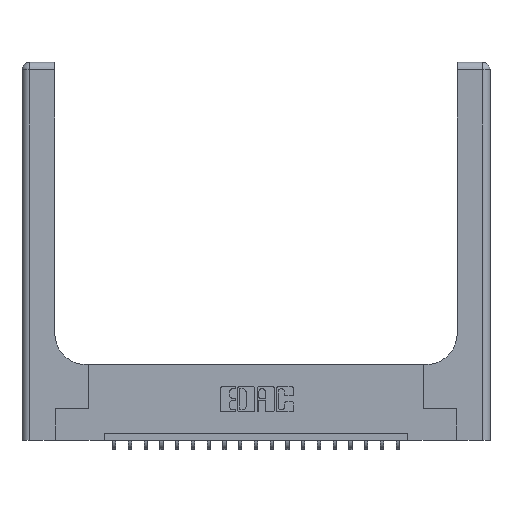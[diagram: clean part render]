
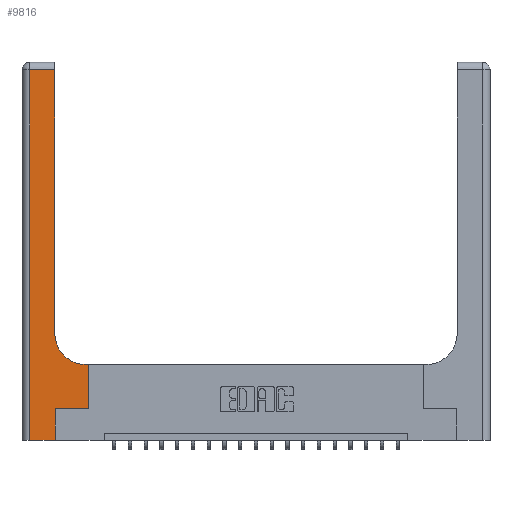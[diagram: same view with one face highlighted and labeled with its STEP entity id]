
A CAD part, top view. The second image highlights one B-rep face of the part: STEP entity #9816.
In plain terms, the highlighted planar face has unit normal (0, 0, 1).
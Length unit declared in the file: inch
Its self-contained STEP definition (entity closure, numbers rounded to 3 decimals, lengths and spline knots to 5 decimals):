
#379 = VERTEX_POINT ( 'NONE', #9639 ) ;
#434 = LINE ( 'NONE', #17205, #19650 ) ;
#571 = AXIS2_PLACEMENT_3D ( 'NONE', #5671, #16478, #7260 ) ;
#612 = VERTEX_POINT ( 'NONE', #17047 ) ;
#637 = VECTOR ( 'NONE', #19210, 39.37008 ) ;
#947 = CARTESIAN_POINT ( 'NONE',  ( 0.265, 0.25, 0.37 ) ) ;
#1096 = CIRCLE ( 'NONE', #571, 0.25 ) ;
#1747 = EDGE_CURVE ( 'NONE', #612, #8378, #14610, .T. ) ;
#2312 = CARTESIAN_POINT ( 'NONE',  ( 0.26, 0.6, 0.37 ) ) ;
#2828 = EDGE_CURVE ( 'NONE', #379, #13615, #1096, .T. ) ;
#3013 = CARTESIAN_POINT ( 'NONE',  ( 0., 0., 0.37 ) ) ;
#3876 = CARTESIAN_POINT ( 'NONE',  ( 0., 3., 0.37 ) ) ;
#3905 = EDGE_CURVE ( 'NONE', #8907, #19641, #17849, .T. ) ;
#3946 = DIRECTION ( 'NONE',  ( -1., 0., 0. ) ) ;
#4446 = EDGE_LOOP ( 'NONE', ( #5739, #5795, #6588, #6672, #7404, #8316, #8670, #9399, #9441 ) ) ;
#4607 = DIRECTION ( 'NONE',  ( 1., 0., 0. ) ) ;
#5671 = CARTESIAN_POINT ( 'NONE',  ( 0.51, 0.85, 0.37 ) ) ;
#5739 = ORIENTED_EDGE ( 'NONE', *, *, #13505, .T. ) ;
#5795 = ORIENTED_EDGE ( 'NONE', *, *, #5980, .T. ) ;
#5980 = EDGE_CURVE ( 'NONE', #20035, #8907, #8693, .T. ) ;
#6588 = ORIENTED_EDGE ( 'NONE', *, *, #3905, .T. ) ;
#6672 = ORIENTED_EDGE ( 'NONE', *, *, #18384, .T. ) ;
#6701 = LINE ( 'NONE', #3013, #14425 ) ;
#6945 = CARTESIAN_POINT ( 'NONE',  ( 0.26, 3., 0.37 ) ) ;
#7023 = DIRECTION ( 'NONE',  ( -1., 0., 0. ) ) ;
#7163 = LINE ( 'NONE', #947, #18428 ) ;
#7234 = CARTESIAN_POINT ( 'NONE',  ( 0.265, 0., 0.37 ) ) ;
#7260 = DIRECTION ( 'NONE',  ( 1., 0., 0. ) ) ;
#7344 = EDGE_CURVE ( 'NONE', #8613, #379, #17656, .T. ) ;
#7404 = ORIENTED_EDGE ( 'NONE', *, *, #1747, .T. ) ;
#8308 = DIRECTION ( 'NONE',  ( 0., -1., 0. ) ) ;
#8316 = ORIENTED_EDGE ( 'NONE', *, *, #13141, .T. ) ;
#8378 = VERTEX_POINT ( 'NONE', #18850 ) ;
#8613 = VERTEX_POINT ( 'NONE', #11750 ) ;
#8670 = ORIENTED_EDGE ( 'NONE', *, *, #18494, .T. ) ;
#8693 = LINE ( 'NONE', #12904, #15411 ) ;
#8907 = VERTEX_POINT ( 'NONE', #18551 ) ;
#9097 = LINE ( 'NONE', #6945, #637 ) ;
#9399 = ORIENTED_EDGE ( 'NONE', *, *, #7344, .T. ) ;
#9441 = ORIENTED_EDGE ( 'NONE', *, *, #2828, .T. ) ;
#9536 = VECTOR ( 'NONE', #3946, 39.37008 ) ;
#9639 = CARTESIAN_POINT ( 'NONE',  ( 0.51, 0.6, 0.37 ) ) ;
#9816 = ADVANCED_FACE ( 'NONE', ( #10890 ), #14703, .F. ) ;
#10423 = CARTESIAN_POINT ( 'NONE',  ( 0.06, 0., 0.37 ) ) ;
#10425 = DIRECTION ( 'NONE',  ( 0., 1., 0. ) ) ;
#10890 = FACE_OUTER_BOUND ( 'NONE', #4446, .T. ) ;
#11750 = CARTESIAN_POINT ( 'NONE',  ( 0.528, 0.6, 0.37 ) ) ;
#12870 = CARTESIAN_POINT ( 'NONE',  ( 0.06, 3., 0.37 ) ) ;
#12904 = CARTESIAN_POINT ( 'NONE',  ( 0., 2.94, 0.37 ) ) ;
#13141 = EDGE_CURVE ( 'NONE', #8378, #16794, #7163, .T. ) ;
#13505 = EDGE_CURVE ( 'NONE', #13615, #20035, #9097, .T. ) ;
#13615 = VERTEX_POINT ( 'NONE', #14888 ) ;
#14425 = VECTOR ( 'NONE', #4607, 39.37008 ) ;
#14470 = DIRECTION ( 'NONE',  ( -1., 0., 0. ) ) ;
#14610 = LINE ( 'NONE', #7234, #18174 ) ;
#14703 = PLANE ( 'NONE',  #17137 ) ;
#14888 = CARTESIAN_POINT ( 'NONE',  ( 0.26, 0.85, 0.37 ) ) ;
#15411 = VECTOR ( 'NONE', #14470, 39.37008 ) ;
#15737 = DIRECTION ( 'NONE',  ( 0., 1., 0. ) ) ;
#16239 = DIRECTION ( 'NONE',  ( 0., 0., -1. ) ) ;
#16478 = DIRECTION ( 'NONE',  ( 0., 0., -1. ) ) ;
#16794 = VERTEX_POINT ( 'NONE', #19940 ) ;
#16904 = VECTOR ( 'NONE', #8308, 39.37008 ) ;
#17047 = CARTESIAN_POINT ( 'NONE',  ( 0.265, 0., 0.37 ) ) ;
#17137 = AXIS2_PLACEMENT_3D ( 'NONE', #3876, #16239, #7023 ) ;
#17205 = CARTESIAN_POINT ( 'NONE',  ( 0.528, 0.25, 0.37 ) ) ;
#17656 = LINE ( 'NONE', #2312, #9536 ) ;
#17849 = LINE ( 'NONE', #12870, #16904 ) ;
#18174 = VECTOR ( 'NONE', #10425, 39.37008 ) ;
#18384 = EDGE_CURVE ( 'NONE', #19641, #612, #6701, .T. ) ;
#18428 = VECTOR ( 'NONE', #19617, 39.37008 ) ;
#18494 = EDGE_CURVE ( 'NONE', #16794, #8613, #434, .T. ) ;
#18551 = CARTESIAN_POINT ( 'NONE',  ( 0.06, 2.94, 0.37 ) ) ;
#18850 = CARTESIAN_POINT ( 'NONE',  ( 0.265, 0.25, 0.37 ) ) ;
#19210 = DIRECTION ( 'NONE',  ( 0., 1., 0. ) ) ;
#19478 = CARTESIAN_POINT ( 'NONE',  ( 0.26, 2.94, 0.37 ) ) ;
#19617 = DIRECTION ( 'NONE',  ( 1., 0., 0. ) ) ;
#19641 = VERTEX_POINT ( 'NONE', #10423 ) ;
#19650 = VECTOR ( 'NONE', #15737, 39.37008 ) ;
#19940 = CARTESIAN_POINT ( 'NONE',  ( 0.528, 0.25, 0.37 ) ) ;
#20035 = VERTEX_POINT ( 'NONE', #19478 ) ;
